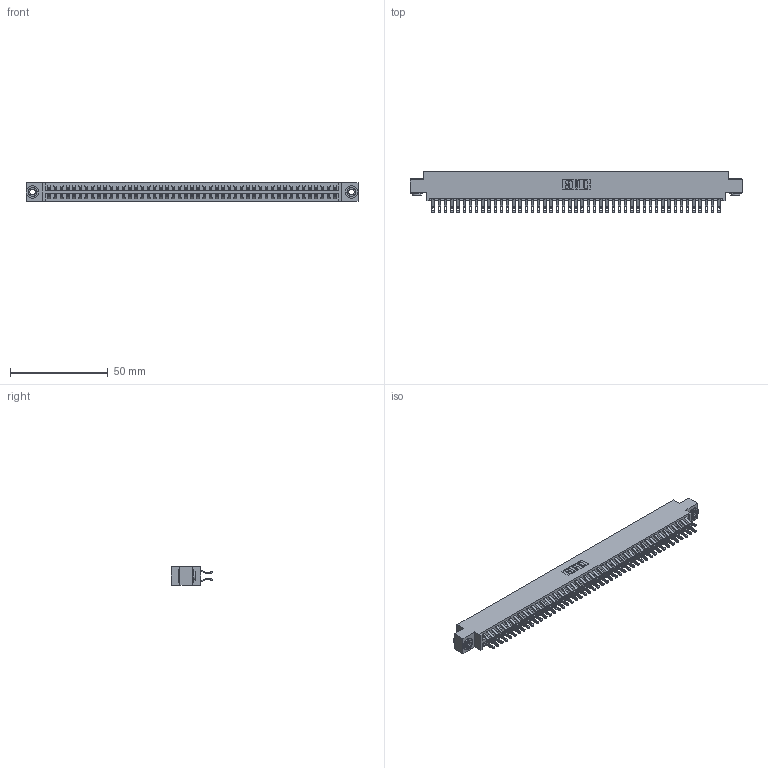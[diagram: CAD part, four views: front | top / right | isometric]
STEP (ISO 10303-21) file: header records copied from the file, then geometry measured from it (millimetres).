
FILE_DESCRIPTION (( 'STEP AP203' ), '1' );
FILE_NAME ('346-094-555-803.STEP', '2022-05-26T14:54:56', ( '' ), ( '' ), 'SwSTEP 2.0', 'SolidWorks 2020', '' );
FILE_SCHEMA (( 'CONFIG_CONTROL_DESIGN' ));
Length unit declared in the file: inch
Products named in the file (4): 346-094-555-803; 345-292-001_555 Tail; 345-250-002_345-250-002-102; 346 Part_0.170 Offset - 0.156 Dia-TH
Assembly tree (97 placements, depth 2):
  346-094-555-803
    346 Part_0.170 Offset - 0.156 Dia-TH
    345-292-001_555 Tail  x94
    345-250-002_345-250-002-102  x2
Bounding box: 169.8 x 21.46 x 9.4 mm (x, y, z)
Volume: 16715.7 mm3; surface area: 24455.7 mm2
Topology: 97 solids, 97 shells, 5630 faces, 17655 edges, 11766 vertices
Faces by surface type: plane 3206, cylinder 2416, cone 8
Entity records: 31524 total; most frequent: CARTESIAN_POINT 5207, ORIENTED_EDGE 5102, DIRECTION 4637, EDGE_CURVE 2551, VECTOR 2187, LINE 2187, VERTEX_POINT 1698, AXIS2_PLACEMENT_3D 1225
